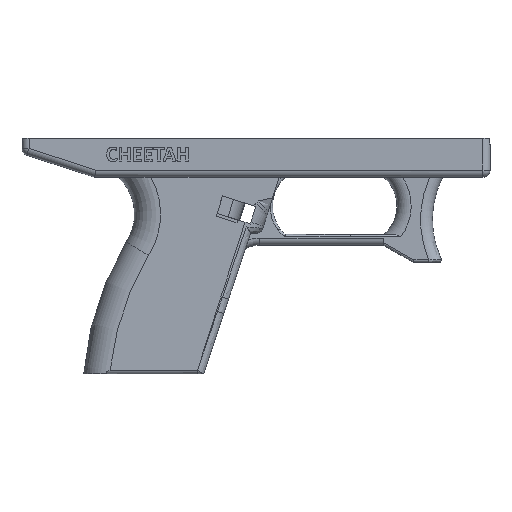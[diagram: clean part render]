
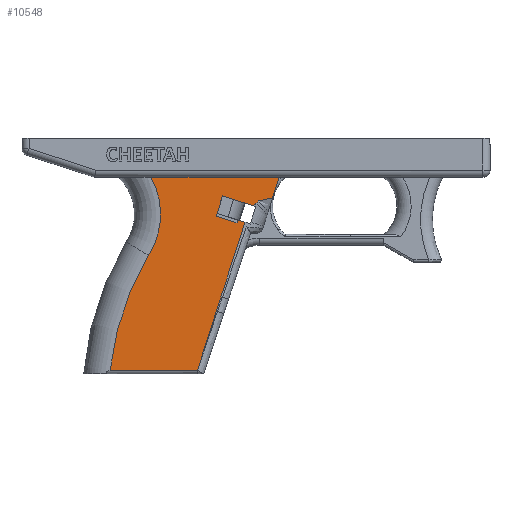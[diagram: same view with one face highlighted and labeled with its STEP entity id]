
A CAD part, front view. The second image highlights one B-rep face of the part: STEP entity #10548.
In plain terms, the highlighted planar face has unit normal (0, -1, 0).
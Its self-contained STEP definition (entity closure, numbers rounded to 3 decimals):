
#231=CIRCLE('',#11053,118.256);
#232=CIRCLE('',#11055,32.243);
#233=CIRCLE('',#11057,18.);
#519=PLANE('',#11056);
#1019=FACE_OUTER_BOUND('',#1600,.T.);
#1600=EDGE_LOOP('',(#9227,#9228,#9229,#9230,#9231,#9232,#9233,#9234,#9235,
#9236,#9237,#9238,#9239,#9240,#9241,#9242,#9243,#9244));
#2168=LINE('',#19146,#3006);
#2169=LINE('',#19147,#3007);
#2278=LINE('',#19652,#3116);
#2360=LINE('',#20225,#3198);
#2361=LINE('',#20227,#3199);
#2364=LINE('',#20295,#3202);
#2418=LINE('',#20670,#3256);
#2419=LINE('',#20671,#3257);
#2420=LINE('',#20673,#3258);
#2421=LINE('',#20675,#3259);
#2422=LINE('',#20677,#3260);
#2423=LINE('',#20679,#3261);
#2424=LINE('',#20681,#3262);
#2425=LINE('',#20685,#3263);
#3006=VECTOR('',#11929,10.);
#3007=VECTOR('',#11930,10.);
#3116=VECTOR('',#12269,10.);
#3198=VECTOR('',#12471,10.);
#3199=VECTOR('',#12472,10.);
#3202=VECTOR('',#12495,10.);
#3256=VECTOR('',#12669,10.);
#3257=VECTOR('',#12670,10.);
#3258=VECTOR('',#12671,10.);
#3259=VECTOR('',#12672,10.);
#3260=VECTOR('',#12673,10.);
#3261=VECTOR('',#12674,10.);
#3262=VECTOR('',#12675,10.);
#3263=VECTOR('',#12678,10.);
#3898=B_SPLINE_CURVE_WITH_KNOTS('',3,(#20686,#20687,#20688,#20689,#20690,
#20691,#20692,#20693),.UNSPECIFIED.,.F.,.F.,(4,2,2,4),(-0.714,
-0.52,0.,0.002),.UNSPECIFIED.);
#4607=VERTEX_POINT('',#19139);
#4608=VERTEX_POINT('',#19143);
#4609=VERTEX_POINT('',#19145);
#4721=VERTEX_POINT('',#19646);
#4722=VERTEX_POINT('',#19651);
#4804=VERTEX_POINT('',#20222);
#4805=VERTEX_POINT('',#20224);
#4806=VERTEX_POINT('',#20226);
#4811=VERTEX_POINT('',#20294);
#4880=VERTEX_POINT('',#20646);
#4881=VERTEX_POINT('',#20653);
#4882=VERTEX_POINT('',#20672);
#4883=VERTEX_POINT('',#20674);
#4884=VERTEX_POINT('',#20676);
#4885=VERTEX_POINT('',#20678);
#4886=VERTEX_POINT('',#20680);
#4887=VERTEX_POINT('',#20682);
#4888=VERTEX_POINT('',#20684);
#5969=EDGE_CURVE('',#4608,#4609,#2168,.T.);
#5970=EDGE_CURVE('',#4609,#4607,#2169,.T.);
#6145=EDGE_CURVE('',#4721,#4722,#2278,.F.);
#6268=EDGE_CURVE('',#4804,#4805,#2360,.T.);
#6269=EDGE_CURVE('',#4805,#4806,#2361,.T.);
#6281=EDGE_CURVE('',#4722,#4811,#2364,.T.);
#6381=EDGE_CURVE('',#4880,#4881,#231,.T.);
#6383=EDGE_CURVE('',#4881,#4721,#232,.T.);
#6384=EDGE_CURVE('',#4607,#4880,#2418,.T.);
#6385=EDGE_CURVE('',#4806,#4608,#2419,.T.);
#6386=EDGE_CURVE('',#4882,#4804,#2420,.T.);
#6387=EDGE_CURVE('',#4883,#4882,#2421,.T.);
#6388=EDGE_CURVE('',#4884,#4883,#2422,.T.);
#6389=EDGE_CURVE('',#4885,#4884,#2423,.T.);
#6390=EDGE_CURVE('',#4886,#4885,#2424,.T.);
#6391=EDGE_CURVE('',#4887,#4886,#233,.T.);
#6392=EDGE_CURVE('',#4888,#4887,#2425,.T.);
#6393=EDGE_CURVE('',#4811,#4888,#3898,.T.);
#9227=ORIENTED_EDGE('',*,*,#6383,.F.);
#9228=ORIENTED_EDGE('',*,*,#6381,.F.);
#9229=ORIENTED_EDGE('',*,*,#6384,.F.);
#9230=ORIENTED_EDGE('',*,*,#5970,.F.);
#9231=ORIENTED_EDGE('',*,*,#5969,.F.);
#9232=ORIENTED_EDGE('',*,*,#6385,.F.);
#9233=ORIENTED_EDGE('',*,*,#6269,.F.);
#9234=ORIENTED_EDGE('',*,*,#6268,.F.);
#9235=ORIENTED_EDGE('',*,*,#6386,.F.);
#9236=ORIENTED_EDGE('',*,*,#6387,.F.);
#9237=ORIENTED_EDGE('',*,*,#6388,.F.);
#9238=ORIENTED_EDGE('',*,*,#6389,.F.);
#9239=ORIENTED_EDGE('',*,*,#6390,.F.);
#9240=ORIENTED_EDGE('',*,*,#6391,.F.);
#9241=ORIENTED_EDGE('',*,*,#6392,.F.);
#9242=ORIENTED_EDGE('',*,*,#6393,.F.);
#9243=ORIENTED_EDGE('',*,*,#6281,.F.);
#9244=ORIENTED_EDGE('',*,*,#6145,.F.);
#10548=ADVANCED_FACE('',(#1019),#519,.F.);
#11053=AXIS2_PLACEMENT_3D('',#20654,#12661,#12662);
#11055=AXIS2_PLACEMENT_3D('',#20668,#12665,#12666);
#11056=AXIS2_PLACEMENT_3D('',#20669,#12667,#12668);
#11057=AXIS2_PLACEMENT_3D('',#20683,#12676,#12677);
#11929=DIRECTION('',(-0.306,0.,-0.952));
#11930=DIRECTION('',(-0.306,0.,-0.952));
#12269=DIRECTION('',(-1.,0.,0.));
#12471=DIRECTION('',(-0.306,0.,-0.952));
#12472=DIRECTION('',(-0.306,0.,-0.952));
#12495=DIRECTION('',(-0.306,0.,-0.952));
#12661=DIRECTION('center_axis',(0.,1.,0.));
#12662=DIRECTION('ref_axis',(-0.952,0.,0.307));
#12665=DIRECTION('center_axis',(0.,-1.,0.));
#12666=DIRECTION('ref_axis',(0.992,0.,0.124));
#12667=DIRECTION('center_axis',(0.,1.,0.));
#12668=DIRECTION('ref_axis',(1.,0.,0.));
#12669=DIRECTION('',(-1.,0.,0.));
#12670=DIRECTION('',(-0.306,0.,-0.952));
#12671=DIRECTION('',(0.952,0.,-0.305));
#12672=DIRECTION('',(0.305,0.,0.952));
#12673=DIRECTION('',(0.952,0.,-0.305));
#12674=DIRECTION('',(-0.305,0.,-0.952));
#12675=DIRECTION('',(-0.952,0.,0.305));
#12676=DIRECTION('center_axis',(0.,-1.,0.));
#12677=DIRECTION('ref_axis',(-0.854,0.,0.521));
#12678=DIRECTION('',(-0.707,0.,-0.707));
#19139=CARTESIAN_POINT('',(102.587,-14.625,-115.82));
#19143=CARTESIAN_POINT('',(110.556,-14.625,-91.));
#19145=CARTESIAN_POINT('',(106.315,-14.625,-104.207));
#19146=CARTESIAN_POINT('',(109.739,-14.625,-93.543));
#19147=CARTESIAN_POINT('',(109.739,-14.625,-93.543));
#19646=CARTESIAN_POINT('',(82.886,-14.625,-34.118));
#19651=CARTESIAN_POINT('',(137.221,-14.625,-34.118));
#19652=CARTESIAN_POINT('',(9.181,-14.625,-34.118));
#20222=CARTESIAN_POINT('',(122.68,-14.625,-53.238));
#20224=CARTESIAN_POINT('',(114.284,-14.625,-79.387));
#20225=CARTESIAN_POINT('',(119.684,-14.625,-62.569));
#20226=CARTESIAN_POINT('',(112.531,-14.625,-84.847));
#20227=CARTESIAN_POINT('',(119.684,-14.625,-62.569));
#20294=CARTESIAN_POINT('',(134.392,-14.625,-42.929));
#20295=CARTESIAN_POINT('',(139.575,-14.625,-26.784));
#20646=CARTESIAN_POINT('',(65.661,-14.625,-115.82));
#20653=CARTESIAN_POINT('',(81.846,-14.625,-67.274));
#20654=CARTESIAN_POINT('Origin',(183.282,-14.625,-128.064));
#20668=CARTESIAN_POINT('Origin',(54.73,-14.625,-49.829));
#20669=CARTESIAN_POINT('Origin',(70.795,-14.625,-75.752));
#20670=CARTESIAN_POINT('',(58.283,-14.625,-115.82));
#20671=CARTESIAN_POINT('',(113.468,-14.625,-81.93));
#20672=CARTESIAN_POINT('',(119.708,-14.625,-52.286));
#20673=CARTESIAN_POINT('',(106.639,-14.625,-48.1));
#20674=CARTESIAN_POINT('',(119.327,-14.625,-53.476));
#20675=CARTESIAN_POINT('',(116.375,-14.625,-62.691));
#20676=CARTESIAN_POINT('',(110.494,-14.625,-50.647));
#20677=CARTESIAN_POINT('',(103.633,-14.625,-48.45));
#20678=CARTESIAN_POINT('',(113.238,-14.625,-42.079));
#20679=CARTESIAN_POINT('',(120.967,-14.625,-17.948));
#20680=CARTESIAN_POINT('',(126.367,-14.625,-46.284));
#20681=CARTESIAN_POINT('',(106.704,-14.625,-39.986));
#20682=CARTESIAN_POINT('',(127.342,-14.625,-45.228));
#20683=CARTESIAN_POINT('Origin',(140.07,-14.625,-57.956));
#20684=CARTESIAN_POINT('',(128.387,-14.625,-44.183));
#20685=CARTESIAN_POINT('',(117.953,-14.625,-54.617));
#20686=CARTESIAN_POINT('Ctrl Pts',(134.392,-14.625,-42.929));
#20687=CARTESIAN_POINT('Ctrl Pts',(133.847,-14.625,-43.055));
#20688=CARTESIAN_POINT('Ctrl Pts',(133.302,-14.625,-43.176));
#20689=CARTESIAN_POINT('Ctrl Pts',(131.31,-14.625,-43.606));
#20690=CARTESIAN_POINT('Ctrl Pts',(130.11,-14.625,-43.844));
#20691=CARTESIAN_POINT('Ctrl Pts',(128.402,-14.625,-44.18));
#20692=CARTESIAN_POINT('Ctrl Pts',(128.394,-14.625,-44.182));
#20693=CARTESIAN_POINT('Ctrl Pts',(128.387,-14.625,-44.183));
